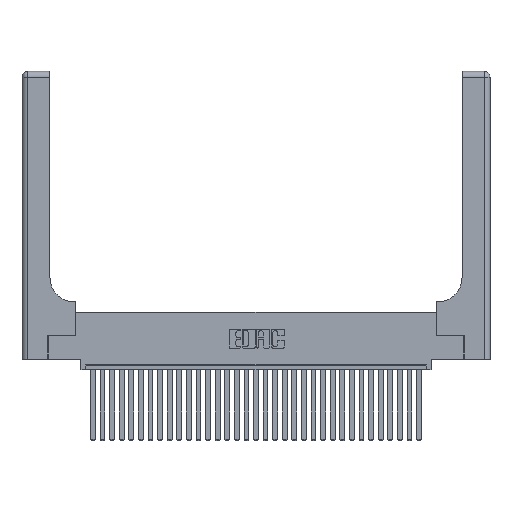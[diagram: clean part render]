
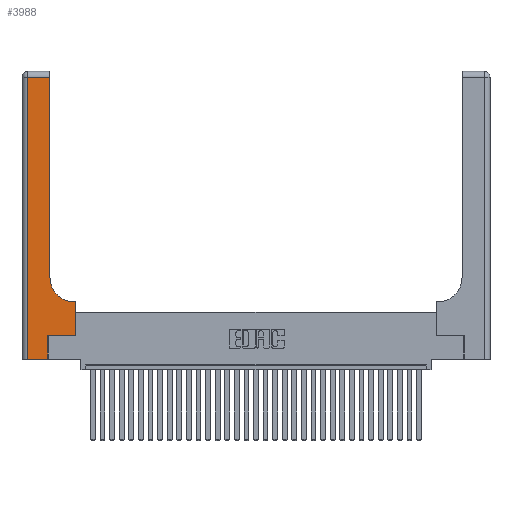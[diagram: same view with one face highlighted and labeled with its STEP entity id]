
A CAD part, top view. The second image highlights one B-rep face of the part: STEP entity #3988.
In plain terms, the highlighted planar face has unit normal (0, 0, 1).
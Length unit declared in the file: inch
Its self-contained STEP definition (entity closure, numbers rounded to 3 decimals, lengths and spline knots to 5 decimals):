
#277 = CARTESIAN_POINT ( 'NONE',  ( 0.269, 0.25, 0.37 ) ) ;
#318 = ORIENTED_EDGE ( 'NONE', *, *, #2498, .T. ) ;
#485 = CARTESIAN_POINT ( 'NONE',  ( 0.269, 0.25, 0.37 ) ) ;
#1370 = VERTEX_POINT ( 'NONE', #3059 ) ;
#1579 = LINE ( 'NONE', #18977, #30186 ) ;
#1777 = VECTOR ( 'NONE', #23940, 39.37008 ) ;
#1841 = EDGE_CURVE ( 'NONE', #5937, #29897, #9123, .T. ) ;
#2498 = EDGE_CURVE ( 'NONE', #5457, #1370, #16145, .T. ) ;
#3059 = CARTESIAN_POINT ( 'NONE',  ( 0.2915, 0.85, 0.37 ) ) ;
#3103 = CARTESIAN_POINT ( 'NONE',  ( 0.5585, 0.25, 0.37 ) ) ;
#3783 = EDGE_CURVE ( 'NONE', #32432, #5937, #25427, .T. ) ;
#3946 = CARTESIAN_POINT ( 'NONE',  ( 0., 2.94, 0.37 ) ) ;
#3988 = ADVANCED_FACE ( 'NONE', ( #16022 ), #22152, .F. ) ;
#4309 = CARTESIAN_POINT ( 'NONE',  ( 0.5415, 0.85, 0.37 ) ) ;
#4516 = CARTESIAN_POINT ( 'NONE',  ( 0.5585, 0.25, 0.37 ) ) ;
#4972 = DIRECTION ( 'NONE',  ( -1., 0., 0. ) ) ;
#5457 = VERTEX_POINT ( 'NONE', #31583 ) ;
#5937 = VERTEX_POINT ( 'NONE', #14469 ) ;
#6037 = DIRECTION ( 'NONE',  ( 0., 1., 0. ) ) ;
#6481 = EDGE_CURVE ( 'NONE', #23200, #24995, #32349, .T. ) ;
#6804 = CARTESIAN_POINT ( 'NONE',  ( 0.269, 0., 0.37 ) ) ;
#7029 = DIRECTION ( 'NONE',  ( -1., 0., 0. ) ) ;
#7610 = VECTOR ( 'NONE', #25352, 39.37008 ) ;
#8933 = CARTESIAN_POINT ( 'NONE',  ( 0.06, 2.94, 0.37 ) ) ;
#9123 = LINE ( 'NONE', #6804, #28277 ) ;
#9173 = LINE ( 'NONE', #9794, #30318 ) ;
#9794 = CARTESIAN_POINT ( 'NONE',  ( 0.2915, 0.6, 0.37 ) ) ;
#9989 = CARTESIAN_POINT ( 'NONE',  ( 0., 3., 0.37 ) ) ;
#10368 = ORIENTED_EDGE ( 'NONE', *, *, #1841, .T. ) ;
#10855 = CARTESIAN_POINT ( 'NONE',  ( 0.5585, 0.6, 0.37 ) ) ;
#11313 = VECTOR ( 'NONE', #27167, 39.37008 ) ;
#11864 = DIRECTION ( 'NONE',  ( 0., 1., 0. ) ) ;
#11992 = DIRECTION ( 'NONE',  ( 1., 0., 0. ) ) ;
#12217 = ORIENTED_EDGE ( 'NONE', *, *, #21322, .T. ) ;
#12223 = EDGE_CURVE ( 'NONE', #24218, #21571, #24879, .T. ) ;
#12403 = LINE ( 'NONE', #277, #7610 ) ;
#13963 = AXIS2_PLACEMENT_3D ( 'NONE', #9989, #17229, #4972 ) ;
#14227 = EDGE_CURVE ( 'NONE', #1370, #23200, #1579, .T. ) ;
#14295 = ORIENTED_EDGE ( 'NONE', *, *, #14227, .T. ) ;
#14403 = CARTESIAN_POINT ( 'NONE',  ( 0., 0., 0.37 ) ) ;
#14469 = CARTESIAN_POINT ( 'NONE',  ( 0.269, 0., 0.37 ) ) ;
#15103 = ORIENTED_EDGE ( 'NONE', *, *, #18934, .T. ) ;
#16022 = FACE_OUTER_BOUND ( 'NONE', #17861, .T. ) ;
#16145 = CIRCLE ( 'NONE', #28147, 0.25 ) ;
#17224 = LINE ( 'NONE', #21848, #11313 ) ;
#17229 = DIRECTION ( 'NONE',  ( 0., 0., -1. ) ) ;
#17632 = ORIENTED_EDGE ( 'NONE', *, *, #12223, .T. ) ;
#17861 = EDGE_LOOP ( 'NONE', ( #14295, #18063, #15103, #23278, #10368, #31620, #17632, #12217, #318 ) ) ;
#18063 = ORIENTED_EDGE ( 'NONE', *, *, #6481, .T. ) ;
#18934 = EDGE_CURVE ( 'NONE', #24995, #32432, #17224, .T. ) ;
#18977 = CARTESIAN_POINT ( 'NONE',  ( 0.2915, 3., 0.37 ) ) ;
#21322 = EDGE_CURVE ( 'NONE', #21571, #5457, #9173, .T. ) ;
#21571 = VERTEX_POINT ( 'NONE', #10855 ) ;
#21848 = CARTESIAN_POINT ( 'NONE',  ( 0.06, 3., 0.37 ) ) ;
#22152 = PLANE ( 'NONE',  #13963 ) ;
#23200 = VERTEX_POINT ( 'NONE', #26445 ) ;
#23278 = ORIENTED_EDGE ( 'NONE', *, *, #3783, .T. ) ;
#23940 = DIRECTION ( 'NONE',  ( -1., 0., 0. ) ) ;
#24218 = VERTEX_POINT ( 'NONE', #4516 ) ;
#24531 = DIRECTION ( 'NONE',  ( 1., 0., 0. ) ) ;
#24879 = LINE ( 'NONE', #3103, #31873 ) ;
#24995 = VERTEX_POINT ( 'NONE', #8933 ) ;
#25352 = DIRECTION ( 'NONE',  ( 1., 0., 0. ) ) ;
#25427 = LINE ( 'NONE', #14403, #32078 ) ;
#25622 = DIRECTION ( 'NONE',  ( 0., 1., 0. ) ) ;
#26445 = CARTESIAN_POINT ( 'NONE',  ( 0.2915, 2.94, 0.37 ) ) ;
#26800 = DIRECTION ( 'NONE',  ( 0., 0., -1. ) ) ;
#27167 = DIRECTION ( 'NONE',  ( 0., -1., 0. ) ) ;
#28118 = EDGE_CURVE ( 'NONE', #29897, #24218, #12403, .T. ) ;
#28147 = AXIS2_PLACEMENT_3D ( 'NONE', #4309, #26800, #24531 ) ;
#28277 = VECTOR ( 'NONE', #11864, 39.37008 ) ;
#29354 = CARTESIAN_POINT ( 'NONE',  ( 0.06, 0., 0.37 ) ) ;
#29897 = VERTEX_POINT ( 'NONE', #485 ) ;
#30186 = VECTOR ( 'NONE', #6037, 39.37008 ) ;
#30318 = VECTOR ( 'NONE', #7029, 39.37008 ) ;
#31583 = CARTESIAN_POINT ( 'NONE',  ( 0.5415, 0.6, 0.37 ) ) ;
#31620 = ORIENTED_EDGE ( 'NONE', *, *, #28118, .T. ) ;
#31873 = VECTOR ( 'NONE', #25622, 39.37008 ) ;
#32078 = VECTOR ( 'NONE', #11992, 39.37008 ) ;
#32349 = LINE ( 'NONE', #3946, #1777 ) ;
#32432 = VERTEX_POINT ( 'NONE', #29354 ) ;
